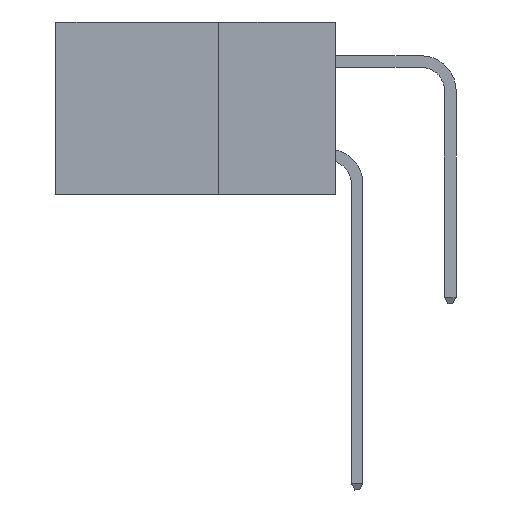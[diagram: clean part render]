
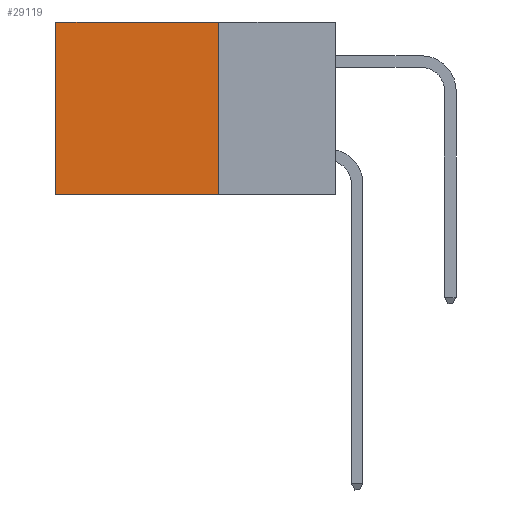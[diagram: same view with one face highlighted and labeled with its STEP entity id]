
A CAD part, left-side view. The second image highlights one B-rep face of the part: STEP entity #29119.
In plain terms, the highlighted planar face has unit normal (-1, 0, 0).
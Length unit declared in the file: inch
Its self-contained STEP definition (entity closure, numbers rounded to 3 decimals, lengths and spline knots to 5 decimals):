
#1109 = LINE ( 'NONE', #13501, #18574 ) ;
#1211 = LINE ( 'NONE', #5889, #15474 ) ;
#2530 = ORIENTED_EDGE ( 'NONE', *, *, #8547, .F. ) ;
#3573 = DIRECTION ( 'NONE',  ( 0., 1., 0. ) ) ;
#3676 = PLANE ( 'NONE',  #25394 ) ;
#3956 = VERTEX_POINT ( 'NONE', #14520 ) ;
#5810 = EDGE_CURVE ( 'NONE', #3956, #26996, #1109, .T. ) ;
#5889 = CARTESIAN_POINT ( 'NONE',  ( 0.2875, 0.25, -0.37 ) ) ;
#7196 = CARTESIAN_POINT ( 'NONE',  ( 0.2875, 0.25, 0. ) ) ;
#8162 = DIRECTION ( 'NONE',  ( 1., 0., 0. ) ) ;
#8547 = EDGE_CURVE ( 'NONE', #23878, #26996, #1211, .T. ) ;
#8567 = CARTESIAN_POINT ( 'NONE',  ( 0.2875, 0.25, -0.37 ) ) ;
#8851 = LINE ( 'NONE', #23369, #12763 ) ;
#9781 = DIRECTION ( 'NONE',  ( 0., 0., -1. ) ) ;
#10748 = DIRECTION ( 'NONE',  ( 0., 0., -1. ) ) ;
#11461 = FACE_OUTER_BOUND ( 'NONE', #25180, .T. ) ;
#12149 = VERTEX_POINT ( 'NONE', #7196 ) ;
#12763 = VECTOR ( 'NONE', #9781, 39.37008 ) ;
#13501 = CARTESIAN_POINT ( 'NONE',  ( 0.2875, 0.6, 0. ) ) ;
#13671 = CARTESIAN_POINT ( 'NONE',  ( 0.2875, 0.25, 0. ) ) ;
#14520 = CARTESIAN_POINT ( 'NONE',  ( 0.2875, 0.6, 0. ) ) ;
#14755 = EDGE_CURVE ( 'NONE', #12149, #3956, #17791, .T. ) ;
#15474 = VECTOR ( 'NONE', #3573, 39.37008 ) ;
#15772 = DIRECTION ( 'NONE',  ( 0., 0., -1. ) ) ;
#16016 = VECTOR ( 'NONE', #17920, 39.37008 ) ;
#16128 = EDGE_CURVE ( 'NONE', #12149, #23878, #8851, .T. ) ;
#17791 = LINE ( 'NONE', #13671, #16016 ) ;
#17920 = DIRECTION ( 'NONE',  ( 0., 1., 0. ) ) ;
#18574 = VECTOR ( 'NONE', #15772, 39.37008 ) ;
#20623 = ORIENTED_EDGE ( 'NONE', *, *, #14755, .T. ) ;
#23123 = CARTESIAN_POINT ( 'NONE',  ( 0.2875, 0.6, -0.37 ) ) ;
#23173 = ORIENTED_EDGE ( 'NONE', *, *, #5810, .T. ) ;
#23369 = CARTESIAN_POINT ( 'NONE',  ( 0.2875, 0.25, 0. ) ) ;
#23878 = VERTEX_POINT ( 'NONE', #8567 ) ;
#25180 = EDGE_LOOP ( 'NONE', ( #23173, #2530, #28673, #20623 ) ) ;
#25394 = AXIS2_PLACEMENT_3D ( 'NONE', #26318, #8162, #10748 ) ;
#26318 = CARTESIAN_POINT ( 'NONE',  ( 0.2875, 0.25, 0. ) ) ;
#26996 = VERTEX_POINT ( 'NONE', #23123 ) ;
#28673 = ORIENTED_EDGE ( 'NONE', *, *, #16128, .F. ) ;
#29119 = ADVANCED_FACE ( 'NONE', ( #11461 ), #3676, .F. ) ;
